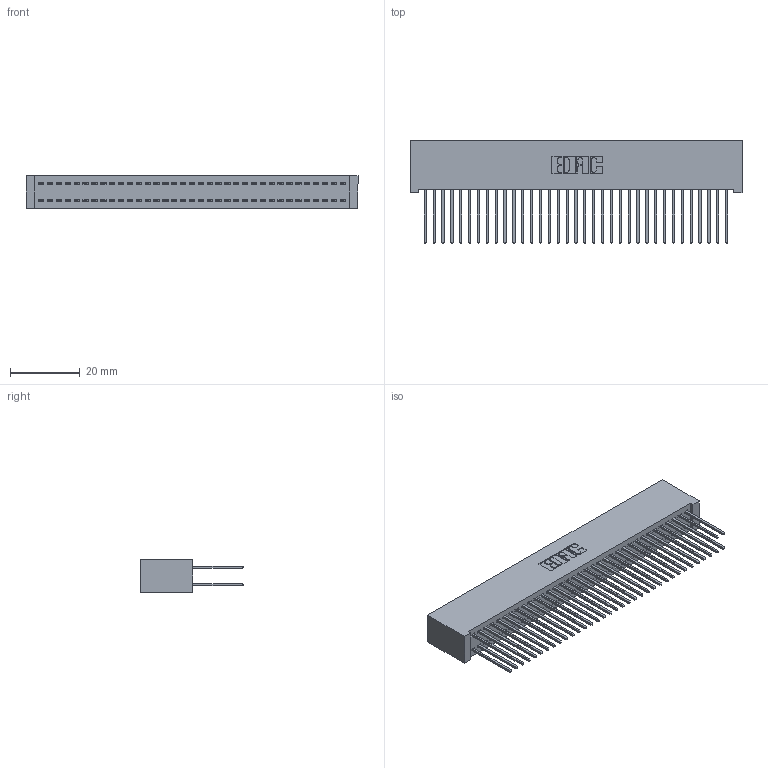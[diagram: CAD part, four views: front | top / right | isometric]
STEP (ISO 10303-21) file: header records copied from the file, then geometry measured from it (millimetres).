
FILE_DESCRIPTION (( 'STEP AP203' ), '1' );
FILE_NAME ('342-070-540-201.STEP', '2018-08-13T09:23:10', ( '' ), ( '' ), 'SwSTEP 2.0', 'SolidWorks 2016', '' );
FILE_SCHEMA (( 'CONFIG_CONTROL_DESIGN' ));
Length unit declared in the file: inch
Products named in the file (3): 342 Part_Lugless; 345-292-001_345-293-140; 342-070-540-201
Assembly tree (71 placements, depth 2):
  342-070-540-201
    342 Part_Lugless
    345-292-001_345-293-140  x70
Bounding box: 95.15 x 29.47 x 9.4 mm (x, y, z)
Volume: 9220.8 mm3; surface area: 16462.6 mm2
Topology: 71 solids, 71 shells, 3742 faces, 11125 edges, 7322 vertices
Faces by surface type: plane 2582, cylinder 1160
Entity records: 23031 total; most frequent: CARTESIAN_POINT 3822, ORIENTED_EDGE 3758, DIRECTION 3271, EDGE_CURVE 1879, VECTOR 1759, LINE 1759, VERTEX_POINT 1250, AXIS2_PLACEMENT_3D 756
